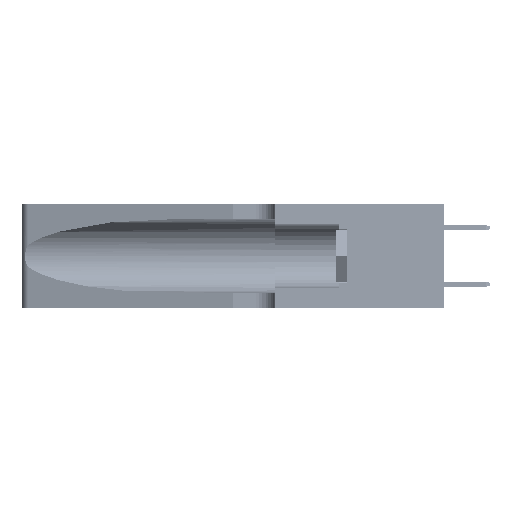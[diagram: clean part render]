
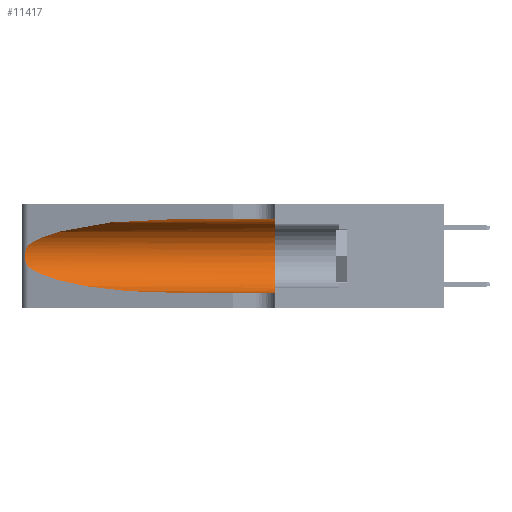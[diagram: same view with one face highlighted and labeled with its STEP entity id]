
A CAD part, left-side view. The second image highlights one B-rep face of the part: STEP entity #11417.
In plain terms, the highlighted cylindrical face has radius 3.308 mm (diameter 6.617 mm), a partial arc.
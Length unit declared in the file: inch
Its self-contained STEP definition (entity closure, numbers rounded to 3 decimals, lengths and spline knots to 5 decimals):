
#180 = CARTESIAN_POINT ( 'NONE',  ( 0.1305, 0.72297, 0.31525 ) ) ;
#225 = DIRECTION ( 'NONE',  ( 0., -1., 0. ) ) ;
#767 = ORIENTED_EDGE ( 'NONE', *, *, #43152, .T. ) ;
#3720 = DIRECTION ( 'NONE',  ( 0., -1., 0. ) ) ;
#5450 = EDGE_CURVE ( 'NONE', #35082, #32446, #30210, .T. ) ;
#7837 = CARTESIAN_POINT ( 'NONE',  ( 0.18966, 0.96281, 0.31525 ) ) ;
#8884 = CYLINDRICAL_SURFACE ( 'NONE', #17468, 0.13025 ) ;
#9360 = ORIENTED_EDGE ( 'NONE', *, *, #11244, .F. ) ;
#10355 = CARTESIAN_POINT ( 'NONE',  ( 0.1305, 0.35, 0.31525 ) ) ;
#10484 = DIRECTION ( 'NONE',  ( 0., -1., 0. ) ) ;
#11244 = EDGE_CURVE ( 'NONE', #17863, #32725, #16076, .T. ) ;
#11387 = DIRECTION ( 'NONE',  ( 0., 0., -1. ) ) ;
#11417 = ADVANCED_FACE ( 'NONE', ( #31632 ), #8884, .F. ) ;
#11529 = CARTESIAN_POINT ( 'NONE',  ( 0.25487, 1.22718, 0.14631 ) ) ;
#12245 = ORIENTED_EDGE ( 'NONE', *, *, #5450, .T. ) ;
#13658 = CARTESIAN_POINT ( 'NONE',  ( 0.25487, 1.22718, 0.14631 ) ) ;
#13808 = CARTESIAN_POINT ( 'NONE',  ( 0.1305, 0.72297, 0.05475 ) ) ;
#14916 = VERTEX_POINT ( 'NONE', #16723 ) ;
#16076 = CIRCLE ( 'NONE', #18438, 0.13025 ) ;
#16723 = CARTESIAN_POINT ( 'NONE',  ( 0.25487, 1.22718, 0.22369 ) ) ;
#17468 = AXIS2_PLACEMENT_3D ( 'NONE', #42347, #225, #11387 ) ;
#17863 = VERTEX_POINT ( 'NONE', #10355 ) ;
#18438 = AXIS2_PLACEMENT_3D ( 'NONE', #20529, #47949, #43780 ) ;
#19165 =( BOUNDED_CURVE ( )  B_SPLINE_CURVE ( 3, ( #180, #7837, #42131, #30931 ),
 .UNSPECIFIED., .F., .T. ) 
 B_SPLINE_CURVE_WITH_KNOTS ( ( 4, 4 ),
 ( 1.5708, 2.84003 ),
 .UNSPECIFIED. ) 
 CURVE ( )  GEOMETRIC_REPRESENTATION_ITEM ( )  RATIONAL_B_SPLINE_CURVE ( ( 1., 0.87, 0.87, 1. ) ) 
 REPRESENTATION_ITEM ( '' )  );
#19218 = CARTESIAN_POINT ( 'NONE',  ( 0.25856, 1.23593, 0.16098 ) ) ;
#19389 = CARTESIAN_POINT ( 'NONE',  ( 0.25487, 1.22718, 0.14631 ) ) ;
#19419 = CARTESIAN_POINT ( 'NONE',  ( 0.1305, 1.61858, 0.31525 ) ) ;
#20073 = EDGE_CURVE ( 'NONE', #14916, #35082, #46467, .T. ) ;
#20529 = CARTESIAN_POINT ( 'NONE',  ( 0.1305, 0.35, 0.185 ) ) ;
#21717 = VERTEX_POINT ( 'NONE', #42897 ) ;
#21951 = CARTESIAN_POINT ( 'NONE',  ( 0.25555, 1.22994, 0.2215 ) ) ;
#22912 = EDGE_CURVE ( 'NONE', #21717, #14916, #19165, .T. ) ;
#26007 = VECTOR ( 'NONE', #3720, 39.37008 ) ;
#26238 = CARTESIAN_POINT ( 'NONE',  ( 0.25854, 1.2359, 0.20912 ) ) ;
#26384 = CARTESIAN_POINT ( 'NONE',  ( 0.25555, 1.22993, 0.14849 ) ) ;
#26531 = ORIENTED_EDGE ( 'NONE', *, *, #22912, .T. ) ;
#29186 = ORIENTED_EDGE ( 'NONE', *, *, #20073, .T. ) ;
#29304 = EDGE_CURVE ( 'NONE', #21717, #17863, #39806, .T. ) ;
#30112 = CARTESIAN_POINT ( 'NONE',  ( 0.26017, 1.23833, 0.17102 ) ) ;
#30210 =( BOUNDED_CURVE ( )  B_SPLINE_CURVE ( 3, ( #13658, #40395, #36710, #13808 ),
 .UNSPECIFIED., .F., .F. ) 
 B_SPLINE_CURVE_WITH_KNOTS ( ( 4, 4 ),
 ( 3.44316, 4.71239 ),
 .UNSPECIFIED. ) 
 CURVE ( )  GEOMETRIC_REPRESENTATION_ITEM ( )  RATIONAL_B_SPLINE_CURVE ( ( 1., 0.87, 0.87, 1. ) ) 
 REPRESENTATION_ITEM ( '' )  );
#30435 = CARTESIAN_POINT ( 'NONE',  ( 0.25639, 1.23186, 0.15144 ) ) ;
#30601 = VECTOR ( 'NONE', #10484, 39.37008 ) ;
#30931 = CARTESIAN_POINT ( 'NONE',  ( 0.25487, 1.22718, 0.22369 ) ) ;
#31373 = ORIENTED_EDGE ( 'NONE', *, *, #29304, .F. ) ;
#31632 = FACE_OUTER_BOUND ( 'NONE', #39137, .T. ) ;
#32446 = VERTEX_POINT ( 'NONE', #47255 ) ;
#32725 = VERTEX_POINT ( 'NONE', #42368 ) ;
#33101 = CARTESIAN_POINT ( 'NONE',  ( 0.1305, 1.61858, 0.05475 ) ) ;
#33970 = CARTESIAN_POINT ( 'NONE',  ( 0.26018, 1.23835, 0.19895 ) ) ;
#34122 = CARTESIAN_POINT ( 'NONE',  ( 0.25789, 1.23486, 0.15765 ) ) ;
#35082 = VERTEX_POINT ( 'NONE', #11529 ) ;
#36710 = CARTESIAN_POINT ( 'NONE',  ( 0.18966, 0.96281, 0.05475 ) ) ;
#38132 = CARTESIAN_POINT ( 'NONE',  ( 0.26075, 1.23896, 0.178 ) ) ;
#39137 = EDGE_LOOP ( 'NONE', ( #26531, #29186, #12245, #767, #9360, #31373 ) ) ;
#39806 = LINE ( 'NONE', #19419, #26007 ) ;
#40395 = CARTESIAN_POINT ( 'NONE',  ( 0.2373, 1.15595, 0.08982 ) ) ;
#42131 = CARTESIAN_POINT ( 'NONE',  ( 0.2373, 1.15595, 0.28018 ) ) ;
#42347 = CARTESIAN_POINT ( 'NONE',  ( 0.1305, 1.61858, 0.185 ) ) ;
#42368 = CARTESIAN_POINT ( 'NONE',  ( 0.1305, 0.35, 0.05475 ) ) ;
#42897 = CARTESIAN_POINT ( 'NONE',  ( 0.1305, 0.72297, 0.31525 ) ) ;
#43152 = EDGE_CURVE ( 'NONE', #32446, #32725, #44961, .T. ) ;
#43780 = DIRECTION ( 'NONE',  ( 0., 0., 1. ) ) ;
#44841 = CARTESIAN_POINT ( 'NONE',  ( 0.25487, 1.22718, 0.22369 ) ) ;
#44961 = LINE ( 'NONE', #33101, #30601 ) ;
#45835 = CARTESIAN_POINT ( 'NONE',  ( 0.25639, 1.23184, 0.21858 ) ) ;
#46154 = CARTESIAN_POINT ( 'NONE',  ( 0.25787, 1.23484, 0.2124 ) ) ;
#46467 = B_SPLINE_CURVE_WITH_KNOTS ( 'NONE', 3,
 ( #44841, #21951, #45835, #46154, #26238, #33970, #49501, #38132, #30112, #19218, #34122, #30435, #26384, #19389 ),
 .UNSPECIFIED., .F., .F.,
 ( 4, 2, 2, 2, 2, 2, 4 ),
 ( 0., 0.00027, 0.00053, 0.00107, 0.0016, 0.00187, 0.00214 ),
 .UNSPECIFIED. ) ;
#47255 = CARTESIAN_POINT ( 'NONE',  ( 0.1305, 0.72297, 0.05475 ) ) ;
#47949 = DIRECTION ( 'NONE',  ( 0., 1., 0. ) ) ;
#49501 = CARTESIAN_POINT ( 'NONE',  ( 0.26075, 1.23896, 0.19203 ) ) ;
